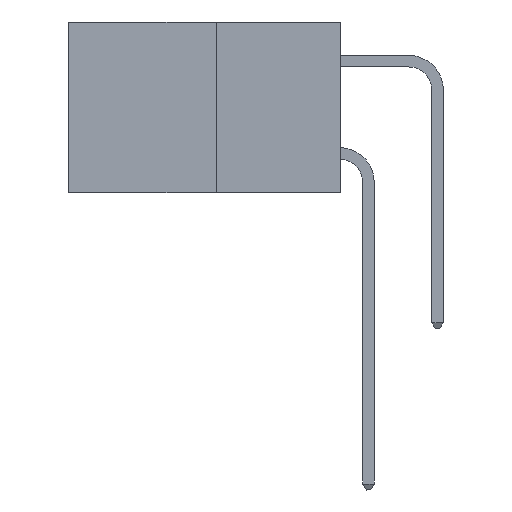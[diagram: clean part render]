
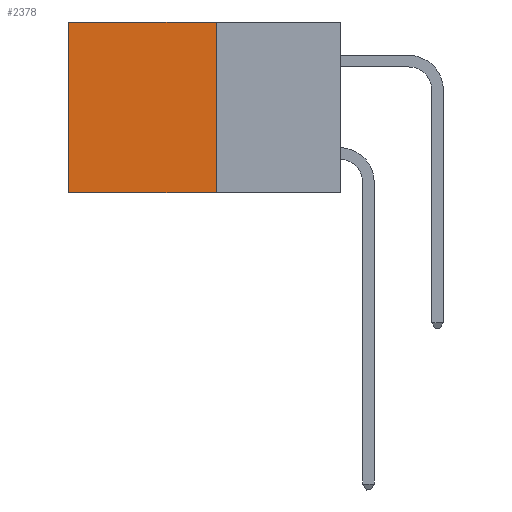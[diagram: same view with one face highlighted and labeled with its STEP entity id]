
A CAD part, left-side view. The second image highlights one B-rep face of the part: STEP entity #2378.
In plain terms, the highlighted planar face has unit normal (-1, 0, 0).
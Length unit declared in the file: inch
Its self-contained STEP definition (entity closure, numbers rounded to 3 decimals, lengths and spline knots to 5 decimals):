
#845 = LINE ( 'NONE', #12833, #9176 ) ;
#975 = CARTESIAN_POINT ( 'NONE',  ( 0.277, 0.27, -0.37 ) ) ;
#1624 = ORIENTED_EDGE ( 'NONE', *, *, #5851, .T. ) ;
#1774 = PLANE ( 'NONE',  #12788 ) ;
#1896 = LINE ( 'NONE', #11512, #12985 ) ;
#2378 = ADVANCED_FACE ( 'NONE', ( #3523 ), #1774, .F. ) ;
#2816 = ORIENTED_EDGE ( 'NONE', *, *, #3467, .F. ) ;
#2931 = CARTESIAN_POINT ( 'NONE',  ( 0.277, 0.27, -0.37 ) ) ;
#3246 = CARTESIAN_POINT ( 'NONE',  ( 0.277, 0.59, -0.37 ) ) ;
#3453 = CARTESIAN_POINT ( 'NONE',  ( 0.277, 0.27, -0.37 ) ) ;
#3467 = EDGE_CURVE ( 'NONE', #6136, #8129, #1896, .T. ) ;
#3523 = FACE_OUTER_BOUND ( 'NONE', #13051, .T. ) ;
#3555 = EDGE_CURVE ( 'NONE', #8462, #8129, #845, .T. ) ;
#3832 = ORIENTED_EDGE ( 'NONE', *, *, #7458, .F. ) ;
#4358 = LINE ( 'NONE', #975, #7256 ) ;
#5851 = EDGE_CURVE ( 'NONE', #10231, #8462, #9775, .T. ) ;
#6136 = VERTEX_POINT ( 'NONE', #2931 ) ;
#6420 = DIRECTION ( 'NONE',  ( 0., 0., -1. ) ) ;
#6936 = VECTOR ( 'NONE', #12203, 39.37008 ) ;
#7059 = CARTESIAN_POINT ( 'NONE',  ( 0.277, 0.27, 0. ) ) ;
#7240 = ORIENTED_EDGE ( 'NONE', *, *, #3555, .T. ) ;
#7256 = VECTOR ( 'NONE', #6420, 39.37008 ) ;
#7458 = EDGE_CURVE ( 'NONE', #10231, #6136, #4358, .T. ) ;
#8007 = CARTESIAN_POINT ( 'NONE',  ( 0.277, 0.59, 0. ) ) ;
#8129 = VERTEX_POINT ( 'NONE', #3246 ) ;
#8462 = VERTEX_POINT ( 'NONE', #8007 ) ;
#9176 = VECTOR ( 'NONE', #12170, 39.37008 ) ;
#9775 = LINE ( 'NONE', #12273, #6936 ) ;
#10231 = VERTEX_POINT ( 'NONE', #7059 ) ;
#10650 = DIRECTION ( 'NONE',  ( 1., 0., 0. ) ) ;
#11512 = CARTESIAN_POINT ( 'NONE',  ( 0.277, 0.27, -0.37 ) ) ;
#12100 = DIRECTION ( 'NONE',  ( 0., 0., -1. ) ) ;
#12170 = DIRECTION ( 'NONE',  ( 0., 0., -1. ) ) ;
#12203 = DIRECTION ( 'NONE',  ( 0., 1., 0. ) ) ;
#12273 = CARTESIAN_POINT ( 'NONE',  ( 0.277, 0.27, 0. ) ) ;
#12788 = AXIS2_PLACEMENT_3D ( 'NONE', #3453, #10650, #12100 ) ;
#12833 = CARTESIAN_POINT ( 'NONE',  ( 0.277, 0.59, -0.37 ) ) ;
#12985 = VECTOR ( 'NONE', #13161, 39.37008 ) ;
#13051 = EDGE_LOOP ( 'NONE', ( #7240, #2816, #3832, #1624 ) ) ;
#13161 = DIRECTION ( 'NONE',  ( 0., 1., 0. ) ) ;
